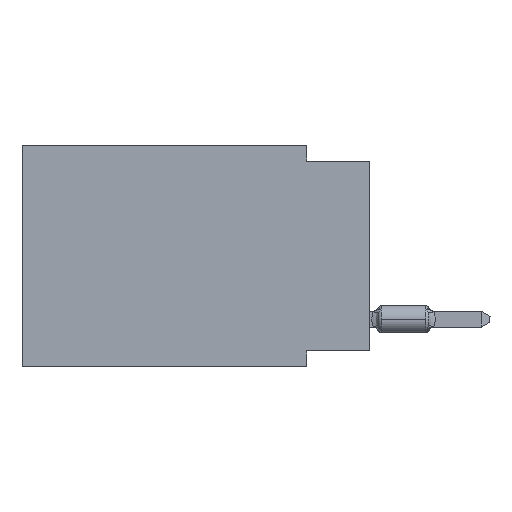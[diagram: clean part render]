
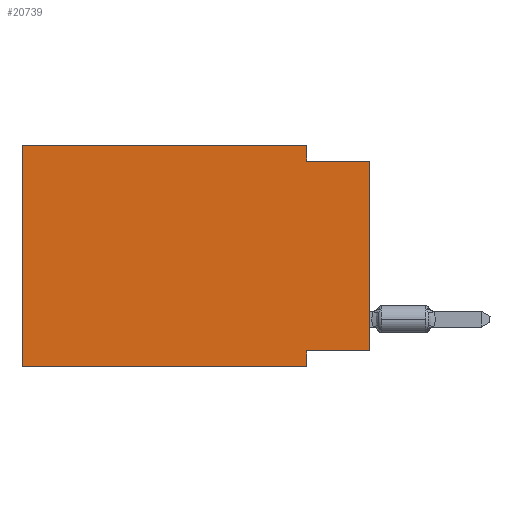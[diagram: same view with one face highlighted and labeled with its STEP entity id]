
A CAD part, left-side view. The second image highlights one B-rep face of the part: STEP entity #20739.
In plain terms, the highlighted planar face has unit normal (-1, 0, 0).
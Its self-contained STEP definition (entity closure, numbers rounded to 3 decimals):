
#167 = LINE ( 'NONE', #25397, #24175 ) ;
#2433 = DIRECTION ( 'NONE',  ( 0., 0., 1. ) ) ;
#2527 = EDGE_CURVE ( 'NONE', #51229, #42435, #7323, .T. ) ;
#3180 = VERTEX_POINT ( 'NONE', #35621 ) ;
#3624 = EDGE_CURVE ( 'NONE', #33574, #3180, #167, .T. ) ;
#4631 = DIRECTION ( 'NONE',  ( 0., 0., -1. ) ) ;
#6387 = VERTEX_POINT ( 'NONE', #24397 ) ;
#7323 = LINE ( 'NONE', #51896, #48601 ) ;
#8447 = DIRECTION ( 'NONE',  ( 0., 0., -1. ) ) ;
#8791 = FACE_OUTER_BOUND ( 'NONE', #25889, .T. ) ;
#9531 = CARTESIAN_POINT ( 'NONE',  ( 0., 2.54, -8.89 ) ) ;
#9695 = CARTESIAN_POINT ( 'NONE',  ( 0., 13.97, 0. ) ) ;
#10487 = VERTEX_POINT ( 'NONE', #26362 ) ;
#12357 = CARTESIAN_POINT ( 'NONE',  ( 0., 0., -0.635 ) ) ;
#12713 = DIRECTION ( 'NONE',  ( 0., 0., -1. ) ) ;
#13060 = CARTESIAN_POINT ( 'NONE',  ( 0., 13.97, 0. ) ) ;
#15904 = DIRECTION ( 'NONE',  ( 0., -1., 0. ) ) ;
#16731 = ORIENTED_EDGE ( 'NONE', *, *, #60139, .F. ) ;
#16912 = ORIENTED_EDGE ( 'NONE', *, *, #51145, .F. ) ;
#17096 = ORIENTED_EDGE ( 'NONE', *, *, #2527, .T. ) ;
#17317 = ORIENTED_EDGE ( 'NONE', *, *, #23814, .F. ) ;
#17977 = CARTESIAN_POINT ( 'NONE',  ( 0., 0., -0.635 ) ) ;
#18213 = VECTOR ( 'NONE', #8447, 1000. ) ;
#20739 = ADVANCED_FACE ( 'NONE', ( #8791 ), #57587, .F. ) ;
#21302 = VECTOR ( 'NONE', #57949, 1000. ) ;
#23814 = EDGE_CURVE ( 'NONE', #51229, #52219, #50213, .T. ) ;
#24175 = VECTOR ( 'NONE', #30005, 1000. ) ;
#24397 = CARTESIAN_POINT ( 'NONE',  ( 0., 13.97, 0. ) ) ;
#24439 = LINE ( 'NONE', #9695, #37814 ) ;
#24808 = CARTESIAN_POINT ( 'NONE',  ( 0., 0., -8.255 ) ) ;
#25397 = CARTESIAN_POINT ( 'NONE',  ( 0., 13.97, -8.89 ) ) ;
#25889 = EDGE_LOOP ( 'NONE', ( #17096, #16731, #16912, #56792, #33268, #35215, #52302, #17317 ) ) ;
#26362 = CARTESIAN_POINT ( 'NONE',  ( 0., 2.54, -0.635 ) ) ;
#27143 = LINE ( 'NONE', #37610, #38053 ) ;
#27826 = CARTESIAN_POINT ( 'NONE',  ( 0., 2.54, -8.255 ) ) ;
#28299 = AXIS2_PLACEMENT_3D ( 'NONE', #13060, #37938, #12713 ) ;
#28435 = CARTESIAN_POINT ( 'NONE',  ( 0., 2.54, 0. ) ) ;
#30005 = DIRECTION ( 'NONE',  ( 0., -1., 0. ) ) ;
#30491 = LINE ( 'NONE', #9531, #56054 ) ;
#31817 = VECTOR ( 'NONE', #60681, 1000. ) ;
#33268 = ORIENTED_EDGE ( 'NONE', *, *, #49026, .F. ) ;
#33574 = VERTEX_POINT ( 'NONE', #63313 ) ;
#35215 = ORIENTED_EDGE ( 'NONE', *, *, #3624, .T. ) ;
#35394 = EDGE_CURVE ( 'NONE', #6387, #64452, #24439, .T. ) ;
#35621 = CARTESIAN_POINT ( 'NONE',  ( 0., 2.54, -8.89 ) ) ;
#37610 = CARTESIAN_POINT ( 'NONE',  ( 0., 13.97, 0. ) ) ;
#37814 = VECTOR ( 'NONE', #15904, 1000. ) ;
#37938 = DIRECTION ( 'NONE',  ( 1., 0., 0. ) ) ;
#38053 = VECTOR ( 'NONE', #47134, 1000. ) ;
#42435 = VERTEX_POINT ( 'NONE', #12357 ) ;
#43538 = LINE ( 'NONE', #17977, #21302 ) ;
#45950 = CARTESIAN_POINT ( 'NONE',  ( 0., 0., -8.255 ) ) ;
#47134 = DIRECTION ( 'NONE',  ( 0., 0., 1. ) ) ;
#47751 = CARTESIAN_POINT ( 'NONE',  ( 0., 2.54, 0. ) ) ;
#48601 = VECTOR ( 'NONE', #2433, 1000. ) ;
#48764 = LINE ( 'NONE', #28435, #18213 ) ;
#49026 = EDGE_CURVE ( 'NONE', #33574, #6387, #27143, .T. ) ;
#50213 = LINE ( 'NONE', #45950, #31817 ) ;
#51145 = EDGE_CURVE ( 'NONE', #64452, #10487, #48764, .T. ) ;
#51229 = VERTEX_POINT ( 'NONE', #24808 ) ;
#51896 = CARTESIAN_POINT ( 'NONE',  ( 0., 0., 0. ) ) ;
#52219 = VERTEX_POINT ( 'NONE', #27826 ) ;
#52302 = ORIENTED_EDGE ( 'NONE', *, *, #64374, .F. ) ;
#56054 = VECTOR ( 'NONE', #4631, 1000. ) ;
#56792 = ORIENTED_EDGE ( 'NONE', *, *, #35394, .F. ) ;
#57587 = PLANE ( 'NONE',  #28299 ) ;
#57949 = DIRECTION ( 'NONE',  ( 0., -1., 0. ) ) ;
#60139 = EDGE_CURVE ( 'NONE', #10487, #42435, #43538, .T. ) ;
#60681 = DIRECTION ( 'NONE',  ( 0., 1., 0. ) ) ;
#63313 = CARTESIAN_POINT ( 'NONE',  ( 0., 13.97, -8.89 ) ) ;
#64374 = EDGE_CURVE ( 'NONE', #52219, #3180, #30491, .T. ) ;
#64452 = VERTEX_POINT ( 'NONE', #47751 ) ;
